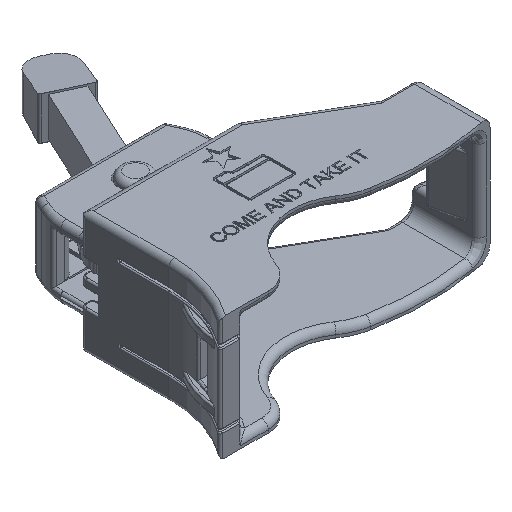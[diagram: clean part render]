
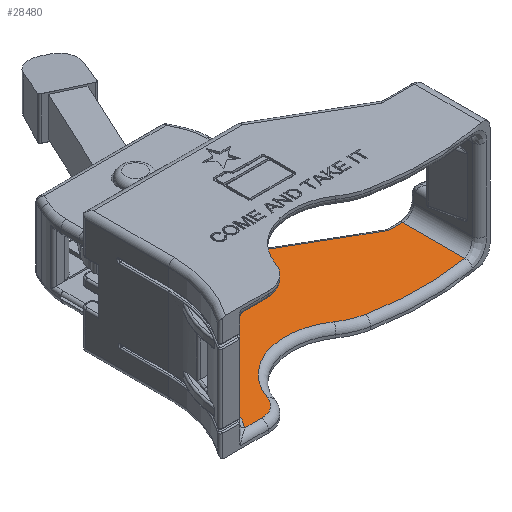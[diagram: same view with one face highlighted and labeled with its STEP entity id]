
A CAD part, isometric view. The second image highlights one B-rep face of the part: STEP entity #28480.
In plain terms, the highlighted planar face has unit normal (0, 0, 1).
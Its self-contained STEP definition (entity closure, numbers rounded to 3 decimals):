
#2522=PLANE('',#29733);
#3823=FACE_OUTER_BOUND('',#5499,.T.);
#5499=EDGE_LOOP('',(#25206,#25207,#25208,#25209,#25210,#25211,#25212,#25213,
#25214,#25215,#25216,#25217,#25218));
#8088=LINE('',#50393,#10740);
#8130=LINE('',#50696,#10782);
#8133=LINE('',#50781,#10785);
#8134=LINE('',#50791,#10786);
#8135=LINE('',#50795,#10787);
#8136=LINE('',#50799,#10788);
#10740=VECTOR('',#34289,10.);
#10782=VECTOR('',#34457,10.);
#10785=VECTOR('',#34486,10.);
#10786=VECTOR('',#34491,10.);
#10787=VECTOR('',#34494,10.);
#10788=VECTOR('',#34497,10.);
#11264=CIRCLE('',#29734,2.);
#11265=CIRCLE('',#29735,2.);
#11266=CIRCLE('',#29736,15.5);
#11267=CIRCLE('',#29737,5.75);
#11268=CIRCLE('',#29738,17.25);
#11269=CIRCLE('',#29739,15.25);
#11270=CIRCLE('',#29740,71.346);
#13786=VERTEX_POINT('',#50376);
#13788=VERTEX_POINT('',#50392);
#13860=VERTEX_POINT('',#50692);
#13869=VERTEX_POINT('',#50780);
#13870=VERTEX_POINT('',#50788);
#13871=VERTEX_POINT('',#50790);
#13872=VERTEX_POINT('',#50792);
#13873=VERTEX_POINT('',#50794);
#13874=VERTEX_POINT('',#50796);
#13875=VERTEX_POINT('',#50798);
#13876=VERTEX_POINT('',#50800);
#13877=VERTEX_POINT('',#50802);
#13878=VERTEX_POINT('',#50804);
#17623=EDGE_CURVE('',#13786,#13788,#8088,.T.);
#17718=EDGE_CURVE('',#13788,#13860,#8130,.T.);
#17732=EDGE_CURVE('',#13860,#13869,#8133,.T.);
#17734=EDGE_CURVE('',#13786,#13870,#11264,.T.);
#17735=EDGE_CURVE('',#13870,#13871,#8134,.F.);
#17736=EDGE_CURVE('',#13872,#13871,#11265,.T.);
#17737=EDGE_CURVE('',#13873,#13872,#8135,.T.);
#17738=EDGE_CURVE('',#13874,#13873,#11266,.T.);
#17739=EDGE_CURVE('',#13875,#13874,#8136,.T.);
#17740=EDGE_CURVE('',#13876,#13875,#11267,.T.);
#17741=EDGE_CURVE('',#13877,#13876,#11268,.T.);
#17742=EDGE_CURVE('',#13878,#13877,#11269,.T.);
#17743=EDGE_CURVE('',#13869,#13878,#11270,.T.);
#25206=ORIENTED_EDGE('',*,*,#17623,.F.);
#25207=ORIENTED_EDGE('',*,*,#17734,.T.);
#25208=ORIENTED_EDGE('',*,*,#17735,.T.);
#25209=ORIENTED_EDGE('',*,*,#17736,.F.);
#25210=ORIENTED_EDGE('',*,*,#17737,.F.);
#25211=ORIENTED_EDGE('',*,*,#17738,.F.);
#25212=ORIENTED_EDGE('',*,*,#17739,.F.);
#25213=ORIENTED_EDGE('',*,*,#17740,.F.);
#25214=ORIENTED_EDGE('',*,*,#17741,.F.);
#25215=ORIENTED_EDGE('',*,*,#17742,.F.);
#25216=ORIENTED_EDGE('',*,*,#17743,.F.);
#25217=ORIENTED_EDGE('',*,*,#17732,.F.);
#25218=ORIENTED_EDGE('',*,*,#17718,.F.);
#28480=ADVANCED_FACE('',(#3823),#2522,.F.);
#29733=AXIS2_PLACEMENT_3D('',#50787,#34487,#34488);
#29734=AXIS2_PLACEMENT_3D('',#50789,#34489,#34490);
#29735=AXIS2_PLACEMENT_3D('',#50793,#34492,#34493);
#29736=AXIS2_PLACEMENT_3D('',#50797,#34495,#34496);
#29737=AXIS2_PLACEMENT_3D('',#50801,#34498,#34499);
#29738=AXIS2_PLACEMENT_3D('',#50803,#34500,#34501);
#29739=AXIS2_PLACEMENT_3D('',#50805,#34502,#34503);
#29740=AXIS2_PLACEMENT_3D('',#50806,#34504,#34505);
#34289=DIRECTION('',(0.866,-0.499,0.));
#34457=DIRECTION('',(1.,0.,0.));
#34486=DIRECTION('',(0.,-1.,0.));
#34487=DIRECTION('center_axis',(0.,0.,-1.));
#34488=DIRECTION('ref_axis',(-1.,0.,0.));
#34489=DIRECTION('center_axis',(0.,0.,-1.));
#34490=DIRECTION('ref_axis',(0.961,0.275,0.));
#34491=DIRECTION('',(1.,0.,0.));
#34492=DIRECTION('center_axis',(0.,0.,1.));
#34493=DIRECTION('ref_axis',(0.917,0.399,0.));
#34494=DIRECTION('',(0.,1.,0.));
#34495=DIRECTION('center_axis',(0.,0.,1.));
#34496=DIRECTION('ref_axis',(0.934,-0.359,0.));
#34497=DIRECTION('',(-1.,0.,0.));
#34498=DIRECTION('center_axis',(0.,0.,-1.));
#34499=DIRECTION('ref_axis',(0.58,-0.814,0.));
#34500=DIRECTION('center_axis',(0.,0.,1.));
#34501=DIRECTION('ref_axis',(-0.311,0.951,0.));
#34502=DIRECTION('center_axis',(0.,0.,-1.));
#34503=DIRECTION('ref_axis',(-0.389,-0.921,0.));
#34504=DIRECTION('center_axis',(0.,0.,-1.));
#34505=DIRECTION('ref_axis',(-0.012,-1.,0.));
#50376=CARTESIAN_POINT('',(38.952,42.054,2.515));
#50392=CARTESIAN_POINT('',(63.522,27.89,2.515));
#50393=CARTESIAN_POINT('',(58.794,30.616,2.515));
#50692=CARTESIAN_POINT('',(67.25,27.89,2.515));
#50696=CARTESIAN_POINT('',(65.375,27.89,2.515));
#50780=CARTESIAN_POINT('',(67.25,11.461,2.515));
#50781=CARTESIAN_POINT('',(67.25,0.,2.515));
#50787=CARTESIAN_POINT('Origin',(68.25,0.,2.515));
#50788=CARTESIAN_POINT('',(37.077,40.75,2.515));
#50789=CARTESIAN_POINT('Origin',(37.077,42.75,2.515));
#50790=CARTESIAN_POINT('',(2.861,40.75,2.515));
#50791=CARTESIAN_POINT('',(51.688,40.75,2.515));
#50792=CARTESIAN_POINT('',(3.,40.018,2.515));
#50793=CARTESIAN_POINT('Origin',(1.,40.018,2.515));
#50794=CARTESIAN_POINT('',(3.,11.456,2.515));
#50795=CARTESIAN_POINT('',(3.,0.,2.515));
#50796=CARTESIAN_POINT('',(-0.416,1.75,2.515));
#50797=CARTESIAN_POINT('Origin',(-12.5,11.456,2.515));
#50798=CARTESIAN_POINT('',(4.007,1.75,2.515));
#50799=CARTESIAN_POINT('',(50.625,1.75,2.515));
#50800=CARTESIAN_POINT('',(9.443,5.625,2.515));
#50801=CARTESIAN_POINT('Origin',(4.007,7.5,2.515));
#50802=CARTESIAN_POINT('',(35.589,14.169,2.515));
#50803=CARTESIAN_POINT('Origin',(25.75,0.,2.515));
#50804=CARTESIAN_POINT('',(41.367,11.727,2.515));
#50805=CARTESIAN_POINT('Origin',(44.287,26.695,2.515));
#50806=CARTESIAN_POINT('Origin',(55.03,81.753,2.515));
